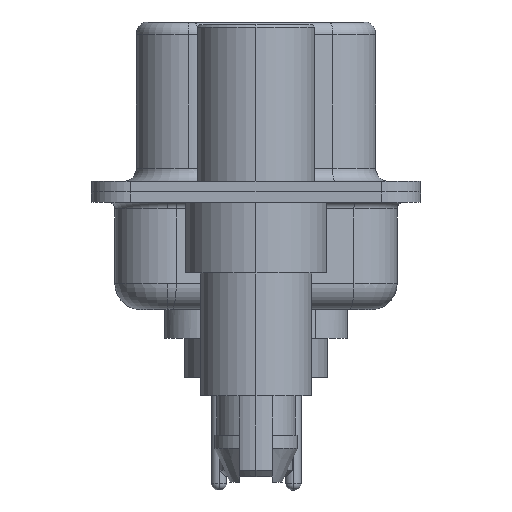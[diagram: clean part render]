
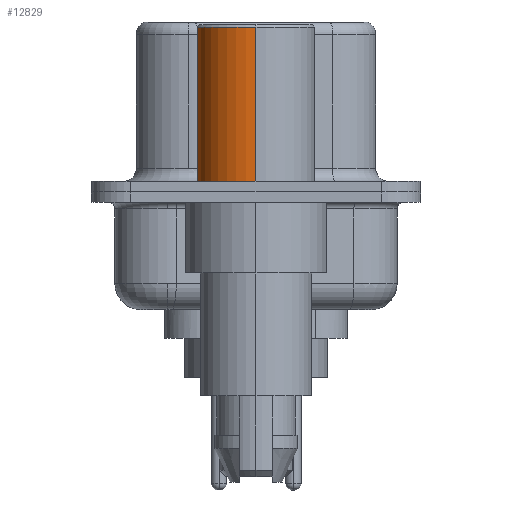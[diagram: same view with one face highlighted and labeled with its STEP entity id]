
A CAD part, left-side view. The second image highlights one B-rep face of the part: STEP entity #12829.
In plain terms, the highlighted cylindrical face has radius 2.25 mm (diameter 4.5 mm), a partial arc.
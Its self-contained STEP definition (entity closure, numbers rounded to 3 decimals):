
#662 = AXIS2_PLACEMENT_3D ( 'NONE', #4053, #14853, #13709 ) ;
#702 = ORIENTED_EDGE ( 'NONE', *, *, #1029, .T. ) ;
#834 = CARTESIAN_POINT ( 'NONE',  ( 0., 0., 0.581 ) ) ;
#1025 = EDGE_CURVE ( 'NONE', #9020, #7553, #3514, .T. ) ;
#1029 = EDGE_CURVE ( 'NONE', #3705, #7553, #11553, .T. ) ;
#1352 = EDGE_CURVE ( 'NONE', #13509, #9020, #5824, .T. ) ;
#1382 = EDGE_CURVE ( 'NONE', #13509, #3705, #12893, .T. ) ;
#2275 = DIRECTION ( 'NONE',  ( 1., 0., 0. ) ) ;
#2618 = ORIENTED_EDGE ( 'NONE', *, *, #1352, .F. ) ;
#2974 = FACE_OUTER_BOUND ( 'NONE', #14797, .T. ) ;
#3514 = CIRCLE ( 'NONE', #662, 2.25 ) ;
#3705 = VERTEX_POINT ( 'NONE', #17871 ) ;
#3727 = DIRECTION ( 'NONE',  ( 0., 0., 1. ) ) ;
#4053 = CARTESIAN_POINT ( 'NONE',  ( 0., 0., 6.3 ) ) ;
#4198 = CARTESIAN_POINT ( 'NONE',  ( -2.25, 0., 6.3 ) ) ;
#4243 = CARTESIAN_POINT ( 'NONE',  ( -2.25, 0., 0.581 ) ) ;
#5517 = ORIENTED_EDGE ( 'NONE', *, *, #1382, .T. ) ;
#5824 = LINE ( 'NONE', #7566, #16465 ) ;
#5868 = ORIENTED_EDGE ( 'NONE', *, *, #1025, .F. ) ;
#5962 = DIRECTION ( 'NONE',  ( 0., 0., 1. ) ) ;
#6115 = CARTESIAN_POINT ( 'NONE',  ( 0., 0., 0.4 ) ) ;
#6182 = DIRECTION ( 'NONE',  ( 0., 0., 1. ) ) ;
#6429 = CYLINDRICAL_SURFACE ( 'NONE', #14473, 2.25 ) ;
#7044 = VECTOR ( 'NONE', #18389, 1000. ) ;
#7553 = VERTEX_POINT ( 'NONE', #4198 ) ;
#7566 = CARTESIAN_POINT ( 'NONE',  ( 2.25, 0., 0.581 ) ) ;
#9020 = VERTEX_POINT ( 'NONE', #12009 ) ;
#11553 = LINE ( 'NONE', #4243, #7044 ) ;
#11858 = DIRECTION ( 'NONE',  ( 1., 0., 0. ) ) ;
#12009 = CARTESIAN_POINT ( 'NONE',  ( 2.25, 0., 6.3 ) ) ;
#12014 = CARTESIAN_POINT ( 'NONE',  ( 2.25, 0., 0.4 ) ) ;
#12829 = ADVANCED_FACE ( 'NONE', ( #2974 ), #6429, .T. ) ;
#12893 = CIRCLE ( 'NONE', #18344, 2.25 ) ;
#13509 = VERTEX_POINT ( 'NONE', #12014 ) ;
#13709 = DIRECTION ( 'NONE',  ( 1., 0., 0. ) ) ;
#14473 = AXIS2_PLACEMENT_3D ( 'NONE', #834, #3727, #2275 ) ;
#14797 = EDGE_LOOP ( 'NONE', ( #5517, #702, #5868, #2618 ) ) ;
#14853 = DIRECTION ( 'NONE',  ( 0., 0., 1. ) ) ;
#16465 = VECTOR ( 'NONE', #5962, 1000. ) ;
#17871 = CARTESIAN_POINT ( 'NONE',  ( -2.25, 0., 0.4 ) ) ;
#18344 = AXIS2_PLACEMENT_3D ( 'NONE', #6115, #6182, #11858 ) ;
#18389 = DIRECTION ( 'NONE',  ( 0., 0., 1. ) ) ;
